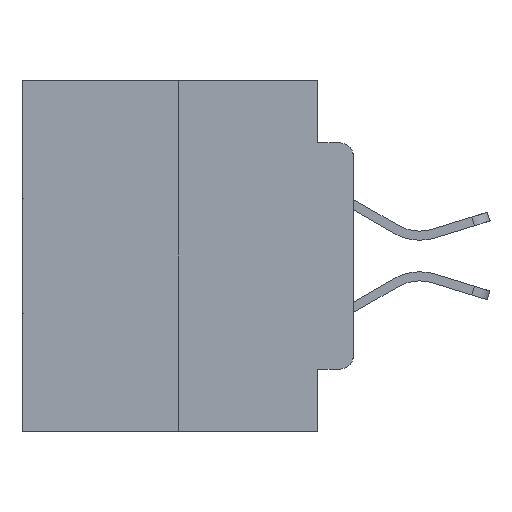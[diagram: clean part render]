
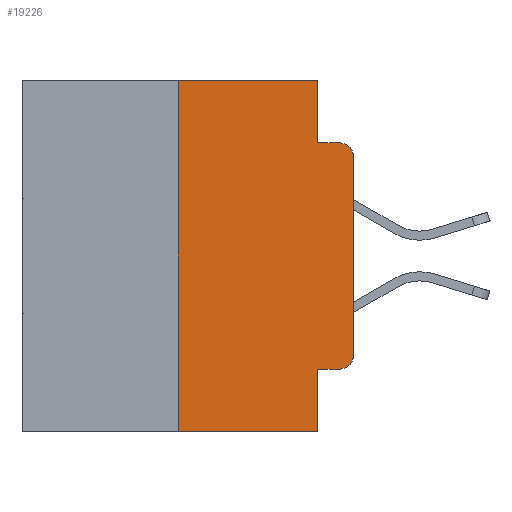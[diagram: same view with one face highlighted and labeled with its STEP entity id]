
A CAD part, left-side view. The second image highlights one B-rep face of the part: STEP entity #19226.
In plain terms, the highlighted planar face has unit normal (-1, 0, 0).
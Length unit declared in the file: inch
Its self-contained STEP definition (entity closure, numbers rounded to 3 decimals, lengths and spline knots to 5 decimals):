
#74 = EDGE_CURVE ( 'NONE', #5012, #17156, #13086, .T. ) ;
#290 = LINE ( 'NONE', #762, #17504 ) ;
#526 = PLANE ( 'NONE',  #21639 ) ;
#762 = CARTESIAN_POINT ( 'NONE',  ( 0., 0.473, -0.5 ) ) ;
#1445 = DIRECTION ( 'NONE',  ( 0., 0., -1. ) ) ;
#1541 = VECTOR ( 'NONE', #2545, 39.37008 ) ;
#1681 = CARTESIAN_POINT ( 'NONE',  ( 0., 0., -0.1085 ) ) ;
#2414 = CARTESIAN_POINT ( 'NONE',  ( 0., 0.25, 0. ) ) ;
#2545 = DIRECTION ( 'NONE',  ( 0., 0., -1. ) ) ;
#3332 = VERTEX_POINT ( 'NONE', #13992 ) ;
#4014 = LINE ( 'NONE', #17079, #9163 ) ;
#4464 = CARTESIAN_POINT ( 'NONE',  ( 0., 0.051, -0.4115 ) ) ;
#4606 = DIRECTION ( 'NONE',  ( 0., 0., 1. ) ) ;
#4780 = VERTEX_POINT ( 'NONE', #1681 ) ;
#4932 = VECTOR ( 'NONE', #26105, 39.37008 ) ;
#5012 = VERTEX_POINT ( 'NONE', #11304 ) ;
#5443 = ORIENTED_EDGE ( 'NONE', *, *, #74, .T. ) ;
#5893 = CARTESIAN_POINT ( 'NONE',  ( 0., 0.02, -0.0885 ) ) ;
#5954 = LINE ( 'NONE', #2414, #16715 ) ;
#6277 = AXIS2_PLACEMENT_3D ( 'NONE', #26880, #14430, #1445 ) ;
#6458 = ORIENTED_EDGE ( 'NONE', *, *, #15805, .F. ) ;
#6746 = VECTOR ( 'NONE', #18259, 39.37008 ) ;
#7074 = CARTESIAN_POINT ( 'NONE',  ( 0., 0.473, 0. ) ) ;
#7130 = ORIENTED_EDGE ( 'NONE', *, *, #7713, .F. ) ;
#7161 = DIRECTION ( 'NONE',  ( 0., 0., -1. ) ) ;
#7171 = EDGE_CURVE ( 'NONE', #16331, #11906, #7342, .T. ) ;
#7342 = LINE ( 'NONE', #26043, #1541 ) ;
#7713 = EDGE_CURVE ( 'NONE', #24648, #3332, #5954, .T. ) ;
#8479 = CARTESIAN_POINT ( 'NONE',  ( 0., 0.051, -0.5 ) ) ;
#8530 = ORIENTED_EDGE ( 'NONE', *, *, #11540, .T. ) ;
#8982 = FACE_OUTER_BOUND ( 'NONE', #9511, .T. ) ;
#9163 = VECTOR ( 'NONE', #19216, 39.37008 ) ;
#9303 = DIRECTION ( 'NONE',  ( 0., 0., -1. ) ) ;
#9511 = EDGE_LOOP ( 'NONE', ( #26915, #11553, #6458, #17884, #23376, #7130, #8530, #20502, #9895, #5443 ) ) ;
#9519 = DIRECTION ( 'NONE',  ( -1., 0., 0. ) ) ;
#9596 = VECTOR ( 'NONE', #25228, 39.37008 ) ;
#9875 = VERTEX_POINT ( 'NONE', #5893 ) ;
#9895 = ORIENTED_EDGE ( 'NONE', *, *, #14576, .T. ) ;
#10274 = CARTESIAN_POINT ( 'NONE',  ( 0., 0.02, -0.3915 ) ) ;
#11249 = VECTOR ( 'NONE', #15596, 39.37008 ) ;
#11304 = CARTESIAN_POINT ( 'NONE',  ( 0., 0.02, -0.4115 ) ) ;
#11475 = CARTESIAN_POINT ( 'NONE',  ( 0., 0., 0. ) ) ;
#11540 = EDGE_CURVE ( 'NONE', #24648, #25799, #290, .T. ) ;
#11553 = ORIENTED_EDGE ( 'NONE', *, *, #17252, .T. ) ;
#11906 = VERTEX_POINT ( 'NONE', #15302 ) ;
#13086 = CIRCLE ( 'NONE', #16511, 0.02 ) ;
#13182 = LINE ( 'NONE', #26527, #6746 ) ;
#13992 = CARTESIAN_POINT ( 'NONE',  ( 0., 0.25, 0. ) ) ;
#14430 = DIRECTION ( 'NONE',  ( -1., 0., 0. ) ) ;
#14576 = EDGE_CURVE ( 'NONE', #21155, #5012, #21498, .T. ) ;
#14830 = CIRCLE ( 'NONE', #6277, 0.02 ) ;
#15007 = CARTESIAN_POINT ( 'NONE',  ( 0., 0.25, -0.5 ) ) ;
#15201 = CARTESIAN_POINT ( 'NONE',  ( 0., 0.051, 0. ) ) ;
#15302 = CARTESIAN_POINT ( 'NONE',  ( 0., 0.051, -0.0885 ) ) ;
#15596 = DIRECTION ( 'NONE',  ( 0., -1., 0. ) ) ;
#15805 = EDGE_CURVE ( 'NONE', #11906, #9875, #22418, .T. ) ;
#15865 = DIRECTION ( 'NONE',  ( 0., -1., 0. ) ) ;
#16331 = VERTEX_POINT ( 'NONE', #15201 ) ;
#16511 = AXIS2_PLACEMENT_3D ( 'NONE', #10274, #9519, #7161 ) ;
#16715 = VECTOR ( 'NONE', #4606, 39.37008 ) ;
#17079 = CARTESIAN_POINT ( 'NONE',  ( 0., 0.051, 0. ) ) ;
#17156 = VERTEX_POINT ( 'NONE', #22373 ) ;
#17252 = EDGE_CURVE ( 'NONE', #4780, #9875, #14830, .T. ) ;
#17504 = VECTOR ( 'NONE', #15865, 39.37008 ) ;
#17884 = ORIENTED_EDGE ( 'NONE', *, *, #7171, .F. ) ;
#18259 = DIRECTION ( 'NONE',  ( 0., -1., 0. ) ) ;
#19216 = DIRECTION ( 'NONE',  ( 0., 0., -1. ) ) ;
#19226 = ADVANCED_FACE ( 'NONE', ( #8982 ), #526, .F. ) ;
#20502 = ORIENTED_EDGE ( 'NONE', *, *, #21586, .F. ) ;
#21155 = VERTEX_POINT ( 'NONE', #4464 ) ;
#21308 = LINE ( 'NONE', #11475, #4932 ) ;
#21498 = LINE ( 'NONE', #27314, #9596 ) ;
#21586 = EDGE_CURVE ( 'NONE', #21155, #25799, #4014, .T. ) ;
#21639 = AXIS2_PLACEMENT_3D ( 'NONE', #7074, #21941, #9303 ) ;
#21914 = CARTESIAN_POINT ( 'NONE',  ( 0., 0.051, -0.0885 ) ) ;
#21941 = DIRECTION ( 'NONE',  ( 1., 0., 0. ) ) ;
#22373 = CARTESIAN_POINT ( 'NONE',  ( 0., 0., -0.3915 ) ) ;
#22418 = LINE ( 'NONE', #21914, #11249 ) ;
#22575 = EDGE_CURVE ( 'NONE', #3332, #16331, #13182, .T. ) ;
#23376 = ORIENTED_EDGE ( 'NONE', *, *, #22575, .F. ) ;
#24184 = EDGE_CURVE ( 'NONE', #17156, #4780, #21308, .T. ) ;
#24648 = VERTEX_POINT ( 'NONE', #15007 ) ;
#25228 = DIRECTION ( 'NONE',  ( 0., -1., 0. ) ) ;
#25799 = VERTEX_POINT ( 'NONE', #8479 ) ;
#26043 = CARTESIAN_POINT ( 'NONE',  ( 0., 0.051, 0. ) ) ;
#26105 = DIRECTION ( 'NONE',  ( 0., 0., 1. ) ) ;
#26527 = CARTESIAN_POINT ( 'NONE',  ( 0., 0.473, 0. ) ) ;
#26880 = CARTESIAN_POINT ( 'NONE',  ( 0., 0.02, -0.1085 ) ) ;
#26915 = ORIENTED_EDGE ( 'NONE', *, *, #24184, .T. ) ;
#27314 = CARTESIAN_POINT ( 'NONE',  ( 0., 0.051, -0.4115 ) ) ;
